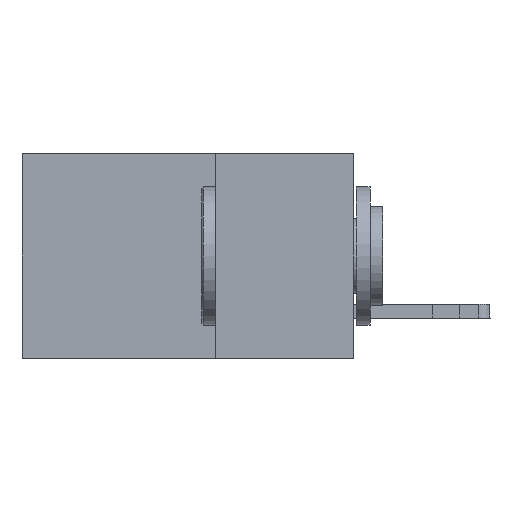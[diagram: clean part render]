
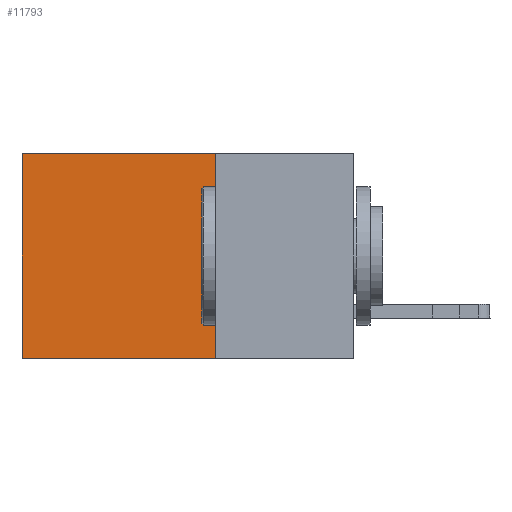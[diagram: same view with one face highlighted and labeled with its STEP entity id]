
A CAD part, left-side view. The second image highlights one B-rep face of the part: STEP entity #11793.
In plain terms, the highlighted planar face has unit normal (-1, 0, 0).
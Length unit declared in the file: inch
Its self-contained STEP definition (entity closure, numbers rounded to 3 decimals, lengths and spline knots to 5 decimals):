
#1806 = DIRECTION ( 'NONE',  ( 1., 0., 0. ) ) ;
#1879 = VECTOR ( 'NONE', #7379, 39.37008 ) ;
#3036 = CARTESIAN_POINT ( 'NONE',  ( 0.2875, 0.25, -0.37 ) ) ;
#3151 = DIRECTION ( 'NONE',  ( 0., 1., 0. ) ) ;
#3884 = CARTESIAN_POINT ( 'NONE',  ( 0.2875, 0.25, 0. ) ) ;
#3903 = CARTESIAN_POINT ( 'NONE',  ( 0.2875, 0.6, 0. ) ) ;
#4072 = DIRECTION ( 'NONE',  ( 0., 0., -1. ) ) ;
#4288 = EDGE_CURVE ( 'NONE', #10355, #14609, #12852, .T. ) ;
#4876 = CARTESIAN_POINT ( 'NONE',  ( 0.2875, 0.25, -0.37 ) ) ;
#5214 = AXIS2_PLACEMENT_3D ( 'NONE', #9599, #1806, #10894 ) ;
#6867 = VECTOR ( 'NONE', #4072, 39.37008 ) ;
#7379 = DIRECTION ( 'NONE',  ( 0., 1., 0. ) ) ;
#8342 = CARTESIAN_POINT ( 'NONE',  ( 0.2875, 0.25, 0. ) ) ;
#8743 = FACE_OUTER_BOUND ( 'NONE', #16012, .T. ) ;
#9016 = DIRECTION ( 'NONE',  ( 0., 0., -1. ) ) ;
#9362 = VERTEX_POINT ( 'NONE', #3903 ) ;
#9599 = CARTESIAN_POINT ( 'NONE',  ( 0.2875, 0.25, 0. ) ) ;
#9806 = LINE ( 'NONE', #12963, #6867 ) ;
#10111 = ORIENTED_EDGE ( 'NONE', *, *, #16266, .T. ) ;
#10355 = VERTEX_POINT ( 'NONE', #4876 ) ;
#10637 = VECTOR ( 'NONE', #9016, 39.37008 ) ;
#10894 = DIRECTION ( 'NONE',  ( 0., 0., -1. ) ) ;
#10916 = ORIENTED_EDGE ( 'NONE', *, *, #4288, .F. ) ;
#11793 = ADVANCED_FACE ( 'NONE', ( #8743 ), #15894, .F. ) ;
#12194 = LINE ( 'NONE', #12344, #1879 ) ;
#12344 = CARTESIAN_POINT ( 'NONE',  ( 0.2875, 0.25, 0. ) ) ;
#12465 = VECTOR ( 'NONE', #3151, 39.37008 ) ;
#12852 = LINE ( 'NONE', #3036, #12465 ) ;
#12963 = CARTESIAN_POINT ( 'NONE',  ( 0.2875, 0.6, 0. ) ) ;
#13027 = VERTEX_POINT ( 'NONE', #8342 ) ;
#14024 = LINE ( 'NONE', #3884, #10637 ) ;
#14336 = EDGE_CURVE ( 'NONE', #13027, #9362, #12194, .T. ) ;
#14609 = VERTEX_POINT ( 'NONE', #15718 ) ;
#15011 = EDGE_CURVE ( 'NONE', #13027, #10355, #14024, .T. ) ;
#15051 = ORIENTED_EDGE ( 'NONE', *, *, #15011, .F. ) ;
#15442 = ORIENTED_EDGE ( 'NONE', *, *, #14336, .T. ) ;
#15718 = CARTESIAN_POINT ( 'NONE',  ( 0.2875, 0.6, -0.37 ) ) ;
#15894 = PLANE ( 'NONE',  #5214 ) ;
#16012 = EDGE_LOOP ( 'NONE', ( #10111, #10916, #15051, #15442 ) ) ;
#16266 = EDGE_CURVE ( 'NONE', #9362, #14609, #9806, .T. ) ;
